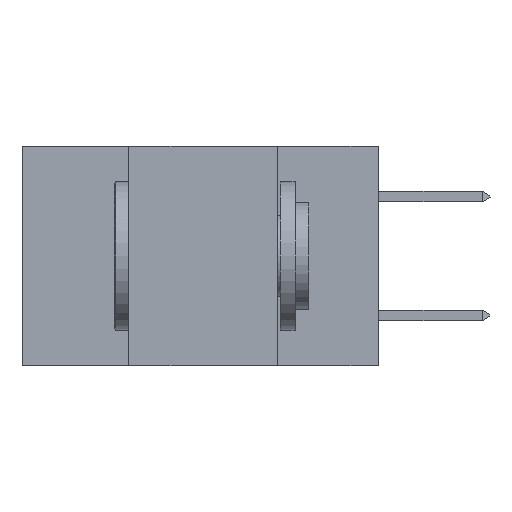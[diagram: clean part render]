
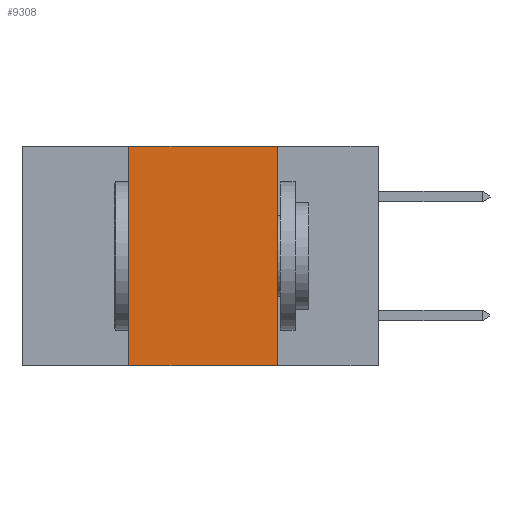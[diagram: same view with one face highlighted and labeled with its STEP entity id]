
A CAD part, left-side view. The second image highlights one B-rep face of the part: STEP entity #9308.
In plain terms, the highlighted planar face has unit normal (-1, 0, 0).
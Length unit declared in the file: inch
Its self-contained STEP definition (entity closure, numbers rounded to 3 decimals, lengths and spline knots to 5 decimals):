
#799 = VERTEX_POINT ( 'NONE', #13437 ) ;
#1065 = CARTESIAN_POINT ( 'NONE',  ( 0., 0.42, 0. ) ) ;
#1572 = CARTESIAN_POINT ( 'NONE',  ( 0., 0.17, 0. ) ) ;
#1955 = CARTESIAN_POINT ( 'NONE',  ( 0., 0.42, -0.37 ) ) ;
#2420 = CARTESIAN_POINT ( 'NONE',  ( 0., 0.6, 0. ) ) ;
#2776 = FACE_OUTER_BOUND ( 'NONE', #12006, .T. ) ;
#4982 = CARTESIAN_POINT ( 'NONE',  ( 0., 0.6, -0.37 ) ) ;
#4998 = ORIENTED_EDGE ( 'NONE', *, *, #12772, .F. ) ;
#5431 = VECTOR ( 'NONE', #17237, 39.37008 ) ;
#5479 = EDGE_CURVE ( 'NONE', #20695, #6526, #19349, .T. ) ;
#5993 = DIRECTION ( 'NONE',  ( 0., 0., -1. ) ) ;
#6526 = VERTEX_POINT ( 'NONE', #14969 ) ;
#6787 = VECTOR ( 'NONE', #5993, 39.37008 ) ;
#7541 = LINE ( 'NONE', #2420, #11661 ) ;
#8806 = DIRECTION ( 'NONE',  ( 1., 0., 0. ) ) ;
#9308 = ADVANCED_FACE ( 'NONE', ( #2776 ), #12270, .F. ) ;
#9569 = VECTOR ( 'NONE', #15041, 39.37008 ) ;
#9615 = ORIENTED_EDGE ( 'NONE', *, *, #9699, .F. ) ;
#9699 = EDGE_CURVE ( 'NONE', #20695, #799, #22359, .T. ) ;
#10975 = AXIS2_PLACEMENT_3D ( 'NONE', #19289, #8806, #21017 ) ;
#11661 = VECTOR ( 'NONE', #14664, 39.37008 ) ;
#12006 = EDGE_LOOP ( 'NONE', ( #13751, #4998, #9615, #14299 ) ) ;
#12270 = PLANE ( 'NONE',  #10975 ) ;
#12772 = EDGE_CURVE ( 'NONE', #799, #18559, #7541, .T. ) ;
#13437 = CARTESIAN_POINT ( 'NONE',  ( 0., 0.42, 0. ) ) ;
#13751 = ORIENTED_EDGE ( 'NONE', *, *, #22100, .F. ) ;
#14299 = ORIENTED_EDGE ( 'NONE', *, *, #5479, .T. ) ;
#14664 = DIRECTION ( 'NONE',  ( 0., -1., 0. ) ) ;
#14969 = CARTESIAN_POINT ( 'NONE',  ( 0., 0.17, -0.37 ) ) ;
#15041 = DIRECTION ( 'NONE',  ( 0., 0., 1. ) ) ;
#16134 = LINE ( 'NONE', #18129, #6787 ) ;
#17237 = DIRECTION ( 'NONE',  ( 0., -1., 0. ) ) ;
#18129 = CARTESIAN_POINT ( 'NONE',  ( 0., 0.17, 0. ) ) ;
#18559 = VERTEX_POINT ( 'NONE', #1572 ) ;
#19289 = CARTESIAN_POINT ( 'NONE',  ( 0., 0.6, 0. ) ) ;
#19349 = LINE ( 'NONE', #4982, #5431 ) ;
#20695 = VERTEX_POINT ( 'NONE', #1955 ) ;
#21017 = DIRECTION ( 'NONE',  ( 0., 0., -1. ) ) ;
#22100 = EDGE_CURVE ( 'NONE', #18559, #6526, #16134, .T. ) ;
#22359 = LINE ( 'NONE', #1065, #9569 ) ;
